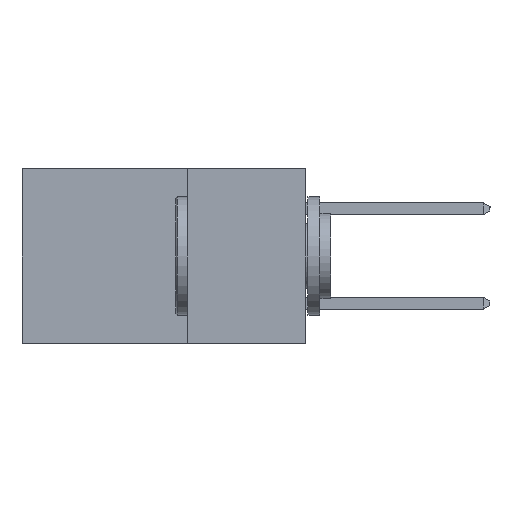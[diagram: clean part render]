
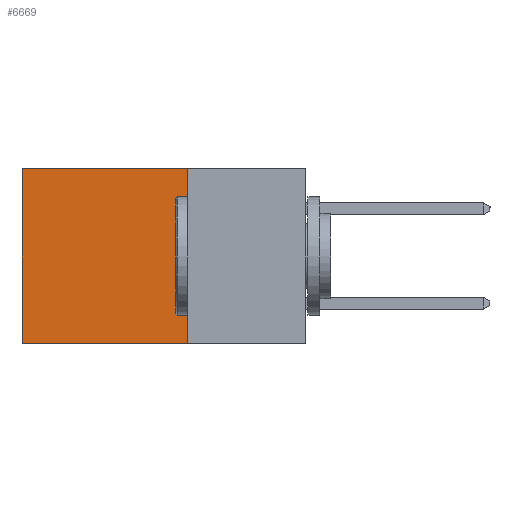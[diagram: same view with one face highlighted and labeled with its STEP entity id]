
A CAD part, left-side view. The second image highlights one B-rep face of the part: STEP entity #6669.
In plain terms, the highlighted planar face has unit normal (-1, 0, 0).
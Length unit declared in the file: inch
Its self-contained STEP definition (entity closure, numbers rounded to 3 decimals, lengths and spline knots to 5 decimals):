
#63 = VECTOR ( 'NONE', #10490, 39.37008 ) ;
#170 = CARTESIAN_POINT ( 'NONE',  ( 0.2615, 0.6, -0.37 ) ) ;
#305 = ORIENTED_EDGE ( 'NONE', *, *, #7396, .T. ) ;
#337 = CARTESIAN_POINT ( 'NONE',  ( 0.2615, 0.25, 0. ) ) ;
#376 = CARTESIAN_POINT ( 'NONE',  ( 0.2615, 0.25, -0.37 ) ) ;
#878 = CARTESIAN_POINT ( 'NONE',  ( 0.2615, 0.6, 0. ) ) ;
#1439 = ORIENTED_EDGE ( 'NONE', *, *, #4426, .F. ) ;
#1509 = VERTEX_POINT ( 'NONE', #10231 ) ;
#1808 = VECTOR ( 'NONE', #9902, 39.37008 ) ;
#2396 = VECTOR ( 'NONE', #4148, 39.37008 ) ;
#2474 = EDGE_CURVE ( 'NONE', #7387, #8585, #8777, .T. ) ;
#2563 = CARTESIAN_POINT ( 'NONE',  ( 0.2615, 0.25, -0.37 ) ) ;
#2860 = LINE ( 'NONE', #170, #7160 ) ;
#3237 = ORIENTED_EDGE ( 'NONE', *, *, #8527, .F. ) ;
#4148 = DIRECTION ( 'NONE',  ( 0., 1., 0. ) ) ;
#4279 = FACE_OUTER_BOUND ( 'NONE', #8574, .T. ) ;
#4383 = DIRECTION ( 'NONE',  ( 0., 0., -1. ) ) ;
#4426 = EDGE_CURVE ( 'NONE', #7387, #7690, #6375, .T. ) ;
#5564 = ORIENTED_EDGE ( 'NONE', *, *, #2474, .T. ) ;
#5923 = DIRECTION ( 'NONE',  ( 1., 0., 0. ) ) ;
#6018 = CARTESIAN_POINT ( 'NONE',  ( 0.2615, 0.25, -0.37 ) ) ;
#6375 = LINE ( 'NONE', #376, #1808 ) ;
#6669 = ADVANCED_FACE ( 'NONE', ( #4279 ), #7799, .F. ) ;
#7140 = DIRECTION ( 'NONE',  ( 0., 0., -1. ) ) ;
#7160 = VECTOR ( 'NONE', #7140, 39.37008 ) ;
#7387 = VERTEX_POINT ( 'NONE', #337 ) ;
#7396 = EDGE_CURVE ( 'NONE', #8585, #1509, #2860, .T. ) ;
#7690 = VERTEX_POINT ( 'NONE', #2563 ) ;
#7799 = PLANE ( 'NONE',  #11137 ) ;
#8527 = EDGE_CURVE ( 'NONE', #7690, #1509, #10166, .T. ) ;
#8574 = EDGE_LOOP ( 'NONE', ( #305, #3237, #1439, #5564 ) ) ;
#8585 = VERTEX_POINT ( 'NONE', #878 ) ;
#8699 = CARTESIAN_POINT ( 'NONE',  ( 0.2615, 0.25, -0.37 ) ) ;
#8777 = LINE ( 'NONE', #10653, #63 ) ;
#9902 = DIRECTION ( 'NONE',  ( 0., 0., -1. ) ) ;
#10166 = LINE ( 'NONE', #6018, #2396 ) ;
#10231 = CARTESIAN_POINT ( 'NONE',  ( 0.2615, 0.6, -0.37 ) ) ;
#10490 = DIRECTION ( 'NONE',  ( 0., 1., 0. ) ) ;
#10653 = CARTESIAN_POINT ( 'NONE',  ( 0.2615, 0.25, 0. ) ) ;
#11137 = AXIS2_PLACEMENT_3D ( 'NONE', #8699, #5923, #4383 ) ;
